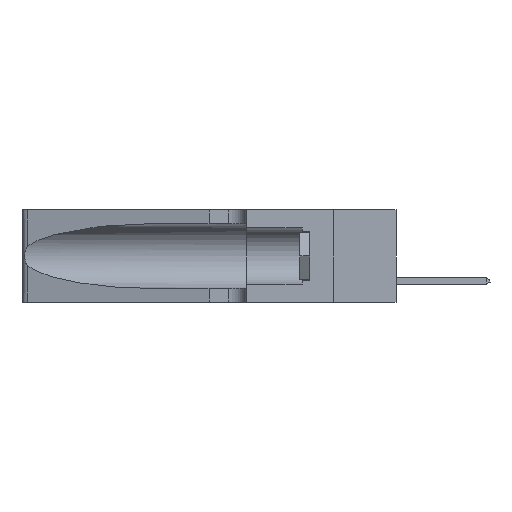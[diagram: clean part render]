
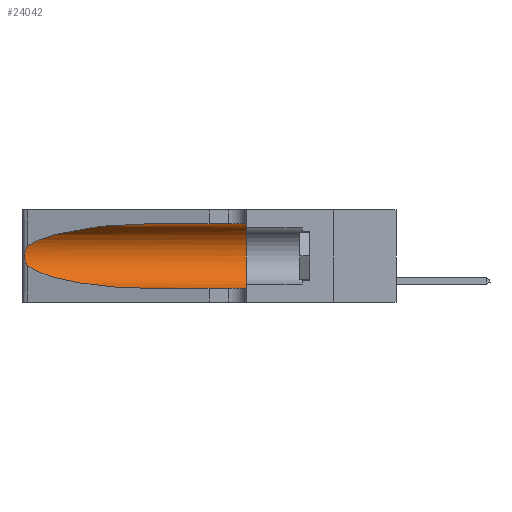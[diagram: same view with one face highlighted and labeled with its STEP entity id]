
A CAD part, left-side view. The second image highlights one B-rep face of the part: STEP entity #24042.
In plain terms, the highlighted cylindrical face has radius 3.308 mm (diameter 6.617 mm), a partial arc.
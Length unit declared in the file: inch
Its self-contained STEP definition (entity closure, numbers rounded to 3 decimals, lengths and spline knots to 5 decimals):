
#332 = VECTOR ( 'NONE', #27871, 39.37008 ) ;
#1431 = CARTESIAN_POINT ( 'NONE',  ( 0.18966, 0.96281, 0.05475 ) ) ;
#3193 = CARTESIAN_POINT ( 'NONE',  ( 0.25555, 1.22994, 0.2215 ) ) ;
#3199 = AXIS2_PLACEMENT_3D ( 'NONE', #19397, #30327, #8689 ) ;
#3354 = CARTESIAN_POINT ( 'NONE',  ( 0.25854, 1.2359, 0.20912 ) ) ;
#3556 = VERTEX_POINT ( 'NONE', #18415 ) ;
#4393 = DIRECTION ( 'NONE',  ( 0., -1., 0. ) ) ;
#4702 = CARTESIAN_POINT ( 'NONE',  ( 0.1305, 1.61858, 0.31525 ) ) ;
#5472 = CIRCLE ( 'NONE', #46280, 0.13025 ) ;
#5644 = CARTESIAN_POINT ( 'NONE',  ( 0.1305, 0.35, 0.185 ) ) ;
#7745 = CARTESIAN_POINT ( 'NONE',  ( 0.26075, 1.23896, 0.178 ) ) ;
#8283 = FACE_OUTER_BOUND ( 'NONE', #18768, .T. ) ;
#8689 = DIRECTION ( 'NONE',  ( 0., 0., -1. ) ) ;
#8803 = DIRECTION ( 'NONE',  ( 0., 1., 0. ) ) ;
#10011 = LINE ( 'NONE', #20137, #332 ) ;
#10799 = VECTOR ( 'NONE', #4393, 39.37008 ) ;
#11500 = CARTESIAN_POINT ( 'NONE',  ( 0.26017, 1.23833, 0.17102 ) ) ;
#12377 = CARTESIAN_POINT ( 'NONE',  ( 0.2373, 1.15595, 0.08982 ) ) ;
#12642 = CARTESIAN_POINT ( 'NONE',  ( 0.25555, 1.22993, 0.14849 ) ) ;
#12888 = CARTESIAN_POINT ( 'NONE',  ( 0.1305, 0.72297, 0.31525 ) ) ;
#13095 = CARTESIAN_POINT ( 'NONE',  ( 0.25487, 1.22718, 0.22369 ) ) ;
#15430 = EDGE_CURVE ( 'NONE', #46545, #33288, #36661, .T. ) ;
#16626 = EDGE_CURVE ( 'NONE', #3556, #37386, #5472, .T. ) ;
#17429 = ORIENTED_EDGE ( 'NONE', *, *, #27891, .T. ) ;
#18025 = CARTESIAN_POINT ( 'NONE',  ( 0.25639, 1.23184, 0.21858 ) ) ;
#18415 = CARTESIAN_POINT ( 'NONE',  ( 0.1305, 0.35, 0.31525 ) ) ;
#18598 = CARTESIAN_POINT ( 'NONE',  ( 0.1305, 0.72297, 0.31525 ) ) ;
#18768 = EDGE_LOOP ( 'NONE', ( #17429, #35666, #38529, #42825, #46666, #39107 ) ) ;
#19397 = CARTESIAN_POINT ( 'NONE',  ( 0.1305, 1.61858, 0.185 ) ) ;
#19693 = CARTESIAN_POINT ( 'NONE',  ( 0.18966, 0.96281, 0.31525 ) ) ;
#20137 = CARTESIAN_POINT ( 'NONE',  ( 0.1305, 1.61858, 0.05475 ) ) ;
#20759 =( BOUNDED_CURVE ( )  B_SPLINE_CURVE ( 3, ( #18598, #19693, #42147, #13095 ),
 .UNSPECIFIED., .F., .T. ) 
 B_SPLINE_CURVE_WITH_KNOTS ( ( 4, 4 ),
 ( 1.5708, 2.84003 ),
 .UNSPECIFIED. ) 
 CURVE ( )  GEOMETRIC_REPRESENTATION_ITEM ( )  RATIONAL_B_SPLINE_CURVE ( ( 1., 0.87, 0.87, 1. ) ) 
 REPRESENTATION_ITEM ( '' )  );
#21178 = CARTESIAN_POINT ( 'NONE',  ( 0.26018, 1.23835, 0.19895 ) ) ;
#22099 = CARTESIAN_POINT ( 'NONE',  ( 0.1305, 0.35, 0.05475 ) ) ;
#22197 = CARTESIAN_POINT ( 'NONE',  ( 0.25856, 1.23593, 0.16098 ) ) ;
#22349 = CARTESIAN_POINT ( 'NONE',  ( 0.25789, 1.23486, 0.15765 ) ) ;
#22454 = CARTESIAN_POINT ( 'NONE',  ( 0.25487, 1.22718, 0.22369 ) ) ;
#22749 = CARTESIAN_POINT ( 'NONE',  ( 0.25487, 1.22718, 0.14631 ) ) ;
#24042 = ADVANCED_FACE ( 'NONE', ( #8283 ), #28033, .F. ) ;
#26277 = EDGE_CURVE ( 'NONE', #33288, #34936, #38390, .T. ) ;
#26681 = EDGE_CURVE ( 'NONE', #35104, #3556, #37316, .T. ) ;
#26714 = CARTESIAN_POINT ( 'NONE',  ( 0.1305, 0.72297, 0.05475 ) ) ;
#27871 = DIRECTION ( 'NONE',  ( 0., -1., 0. ) ) ;
#27891 = EDGE_CURVE ( 'NONE', #35104, #46545, #20759, .T. ) ;
#28033 = CYLINDRICAL_SURFACE ( 'NONE', #3199, 0.13025 ) ;
#29046 = CARTESIAN_POINT ( 'NONE',  ( 0.25787, 1.23484, 0.2124 ) ) ;
#30327 = DIRECTION ( 'NONE',  ( 0., -1., 0. ) ) ;
#30446 = DIRECTION ( 'NONE',  ( 0., 0., 1. ) ) ;
#31020 = CARTESIAN_POINT ( 'NONE',  ( 0.25487, 1.22718, 0.14631 ) ) ;
#31253 = CARTESIAN_POINT ( 'NONE',  ( 0.25487, 1.22718, 0.14631 ) ) ;
#33288 = VERTEX_POINT ( 'NONE', #31020 ) ;
#34099 = CARTESIAN_POINT ( 'NONE',  ( 0.26075, 1.23896, 0.19203 ) ) ;
#34936 = VERTEX_POINT ( 'NONE', #35533 ) ;
#35104 = VERTEX_POINT ( 'NONE', #12888 ) ;
#35533 = CARTESIAN_POINT ( 'NONE',  ( 0.1305, 0.72297, 0.05475 ) ) ;
#35666 = ORIENTED_EDGE ( 'NONE', *, *, #15430, .T. ) ;
#36661 = B_SPLINE_CURVE_WITH_KNOTS ( 'NONE', 3,
 ( #43127, #3193, #18025, #29046, #3354, #21178, #34099, #7745, #11500, #22197, #22349, #37569, #12642, #31253 ),
 .UNSPECIFIED., .F., .F.,
 ( 4, 2, 2, 2, 2, 2, 4 ),
 ( 0., 0.00027, 0.00053, 0.00107, 0.0016, 0.00187, 0.00214 ),
 .UNSPECIFIED. ) ;
#37316 = LINE ( 'NONE', #4702, #10799 ) ;
#37386 = VERTEX_POINT ( 'NONE', #22099 ) ;
#37569 = CARTESIAN_POINT ( 'NONE',  ( 0.25639, 1.23186, 0.15144 ) ) ;
#38390 =( BOUNDED_CURVE ( )  B_SPLINE_CURVE ( 3, ( #22749, #12377, #1431, #26714 ),
 .UNSPECIFIED., .F., .F. ) 
 B_SPLINE_CURVE_WITH_KNOTS ( ( 4, 4 ),
 ( 3.44316, 4.71239 ),
 .UNSPECIFIED. ) 
 CURVE ( )  GEOMETRIC_REPRESENTATION_ITEM ( )  RATIONAL_B_SPLINE_CURVE ( ( 1., 0.87, 0.87, 1. ) ) 
 REPRESENTATION_ITEM ( '' )  );
#38529 = ORIENTED_EDGE ( 'NONE', *, *, #26277, .T. ) ;
#39107 = ORIENTED_EDGE ( 'NONE', *, *, #26681, .F. ) ;
#39984 = EDGE_CURVE ( 'NONE', #34936, #37386, #10011, .T. ) ;
#42147 = CARTESIAN_POINT ( 'NONE',  ( 0.2373, 1.15595, 0.28018 ) ) ;
#42825 = ORIENTED_EDGE ( 'NONE', *, *, #39984, .T. ) ;
#43127 = CARTESIAN_POINT ( 'NONE',  ( 0.25487, 1.22718, 0.22369 ) ) ;
#46280 = AXIS2_PLACEMENT_3D ( 'NONE', #5644, #8803, #30446 ) ;
#46545 = VERTEX_POINT ( 'NONE', #22454 ) ;
#46666 = ORIENTED_EDGE ( 'NONE', *, *, #16626, .F. ) ;
